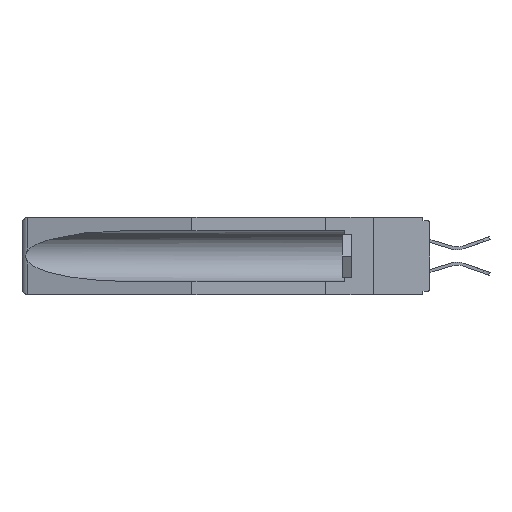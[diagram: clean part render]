
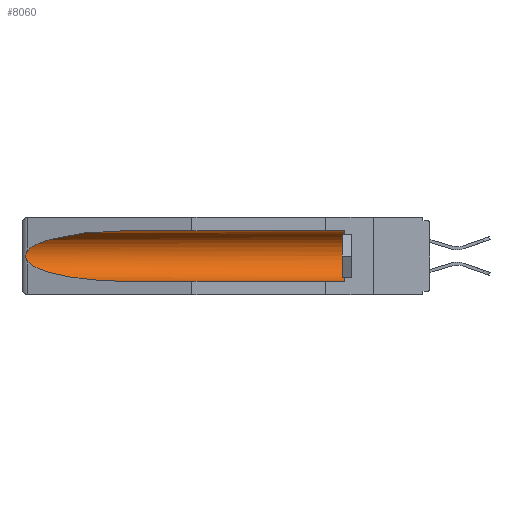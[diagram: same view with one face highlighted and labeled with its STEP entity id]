
A CAD part, left-side view. The second image highlights one B-rep face of the part: STEP entity #8060.
In plain terms, the highlighted cylindrical face has radius 2.857 mm (diameter 5.715 mm), a partial arc.
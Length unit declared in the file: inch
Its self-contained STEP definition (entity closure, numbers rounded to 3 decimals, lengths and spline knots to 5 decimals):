
#760 = CARTESIAN_POINT ( 'NONE',  ( 0.155, 1.07973, -0.059 ) ) ;
#1066 = EDGE_CURVE ( 'NONE', #5734, #5303, #21743, .T. ) ;
#1466 = B_SPLINE_CURVE_WITH_KNOTS ( 'NONE', 3,
 ( #27650, #20609, #22734, #22942, #6722, #8771, #11321, #1929, #9079, #29815 ),
 .UNSPECIFIED., .F., .F.,
 ( 4, 2, 2, 2, 4 ),
 ( 0., 0.00029, 0.00058, 0.00087, 0.00117 ),
 .UNSPECIFIED. ) ;
#1504 = EDGE_CURVE ( 'NONE', #16624, #14132, #22618, .T. ) ;
#1614 = DIRECTION ( 'NONE',  ( 0., 1., 0. ) ) ;
#1929 = CARTESIAN_POINT ( 'NONE',  ( 0.26655, 1.53094, -0.18657 ) ) ;
#2790 = CARTESIAN_POINT ( 'NONE',  ( 0.26537, 1.52718, -0.14972 ) ) ;
#3173 = CARTESIAN_POINT ( 'NONE',  ( 0.26537, 1.52718, -0.19328 ) ) ;
#3912 = EDGE_CURVE ( 'NONE', #19961, #5734, #8403, .T. ) ;
#4807 = CARTESIAN_POINT ( 'NONE',  ( 0.26537, 1.52718, -0.19328 ) ) ;
#5166 = EDGE_CURVE ( 'NONE', #19964, #16624, #1466, .T. ) ;
#5303 = VERTEX_POINT ( 'NONE', #760 ) ;
#5704 = EDGE_CURVE ( 'NONE', #5303, #19964, #9924, .T. ) ;
#5734 = VERTEX_POINT ( 'NONE', #8223 ) ;
#5757 = DIRECTION ( 'NONE',  ( 0., 0., 1. ) ) ;
#6722 = CARTESIAN_POINT ( 'NONE',  ( 0.2675, 1.53308, -0.16763 ) ) ;
#6724 = DIRECTION ( 'NONE',  ( 0., 0., 1. ) ) ;
#6966 = EDGE_CURVE ( 'NONE', #19961, #14132, #21875, .T. ) ;
#7231 = CARTESIAN_POINT ( 'NONE',  ( 0.21114, 1.30732, -0.059 ) ) ;
#8060 = ADVANCED_FACE ( 'NONE', ( #22507 ), #10118, .F. ) ;
#8223 = CARTESIAN_POINT ( 'NONE',  ( 0.155, 0.126, -0.059 ) ) ;
#8403 = CIRCLE ( 'NONE', #21635, 0.1125 ) ;
#8771 = CARTESIAN_POINT ( 'NONE',  ( 0.2675, 1.53308, -0.17534 ) ) ;
#9065 = DIRECTION ( 'NONE',  ( 0., 1., 0. ) ) ;
#9079 = CARTESIAN_POINT ( 'NONE',  ( 0.26597, 1.5296, -0.19026 ) ) ;
#9643 = CARTESIAN_POINT ( 'NONE',  ( 0.25451, 1.48313, -0.24835 ) ) ;
#9924 =( BOUNDED_CURVE ( )  B_SPLINE_CURVE ( 3, ( #13668, #7231, #25914, #14076 ),
 .UNSPECIFIED., .F., .F. ) 
 B_SPLINE_CURVE_WITH_KNOTS ( ( 4, 4 ),
 ( 4.71239, 6.08839 ),
 .UNSPECIFIED. ) 
 CURVE ( )  GEOMETRIC_REPRESENTATION_ITEM ( )  RATIONAL_B_SPLINE_CURVE ( ( 1., 0.848, 0.848, 1. ) ) 
 REPRESENTATION_ITEM ( '' )  );
#10118 = CYLINDRICAL_SURFACE ( 'NONE', #18815, 0.1125 ) ;
#11321 = CARTESIAN_POINT ( 'NONE',  ( 0.2673, 1.53269, -0.17917 ) ) ;
#12942 = DIRECTION ( 'NONE',  ( 0., 1., 0. ) ) ;
#13277 = ORIENTED_EDGE ( 'NONE', *, *, #1504, .T. ) ;
#13668 = CARTESIAN_POINT ( 'NONE',  ( 0.155, 1.07973, -0.059 ) ) ;
#13702 = VECTOR ( 'NONE', #9065, 39.37008 ) ;
#14076 = CARTESIAN_POINT ( 'NONE',  ( 0.26537, 1.52718, -0.14972 ) ) ;
#14132 = VERTEX_POINT ( 'NONE', #18779 ) ;
#14437 = CARTESIAN_POINT ( 'NONE',  ( 0.155, 1.07973, -0.284 ) ) ;
#14639 = ORIENTED_EDGE ( 'NONE', *, *, #1066, .T. ) ;
#15989 = CARTESIAN_POINT ( 'NONE',  ( 0.155, -0.30754, -0.059 ) ) ;
#16254 = ORIENTED_EDGE ( 'NONE', *, *, #5166, .T. ) ;
#16589 = CARTESIAN_POINT ( 'NONE',  ( 0.155, 0.126, -0.284 ) ) ;
#16624 = VERTEX_POINT ( 'NONE', #3173 ) ;
#18779 = CARTESIAN_POINT ( 'NONE',  ( 0.155, 1.07973, -0.284 ) ) ;
#18815 = AXIS2_PLACEMENT_3D ( 'NONE', #25103, #1614, #6724 ) ;
#19131 = CARTESIAN_POINT ( 'NONE',  ( 0.155, -0.30754, -0.284 ) ) ;
#19487 = ORIENTED_EDGE ( 'NONE', *, *, #3912, .T. ) ;
#19795 = CARTESIAN_POINT ( 'NONE',  ( 0.155, 0.126, -0.1715 ) ) ;
#19961 = VERTEX_POINT ( 'NONE', #16589 ) ;
#19964 = VERTEX_POINT ( 'NONE', #2790 ) ;
#20609 = CARTESIAN_POINT ( 'NONE',  ( 0.26597, 1.52961, -0.15275 ) ) ;
#21169 = CARTESIAN_POINT ( 'NONE',  ( 0.21114, 1.30732, -0.284 ) ) ;
#21635 = AXIS2_PLACEMENT_3D ( 'NONE', #19795, #21798, #5757 ) ;
#21743 = LINE ( 'NONE', #15989, #13702 ) ;
#21798 = DIRECTION ( 'NONE',  ( 0., -1., 0. ) ) ;
#21875 = LINE ( 'NONE', #19131, #27733 ) ;
#22507 = FACE_OUTER_BOUND ( 'NONE', #24302, .T. ) ;
#22618 =( BOUNDED_CURVE ( )  B_SPLINE_CURVE ( 3, ( #4807, #9643, #21169, #14437 ),
 .UNSPECIFIED., .F., .F. ) 
 B_SPLINE_CURVE_WITH_KNOTS ( ( 4, 4 ),
 ( 0.1948, 1.5708 ),
 .UNSPECIFIED. ) 
 CURVE ( )  GEOMETRIC_REPRESENTATION_ITEM ( )  RATIONAL_B_SPLINE_CURVE ( ( 1., 0.848, 0.848, 1. ) ) 
 REPRESENTATION_ITEM ( '' )  );
#22734 = CARTESIAN_POINT ( 'NONE',  ( 0.26654, 1.53092, -0.15636 ) ) ;
#22942 = CARTESIAN_POINT ( 'NONE',  ( 0.2673, 1.5327, -0.16383 ) ) ;
#24302 = EDGE_LOOP ( 'NONE', ( #26652, #16254, #13277, #28829, #19487, #14639 ) ) ;
#25103 = CARTESIAN_POINT ( 'NONE',  ( 0.155, -0.30754, -0.1715 ) ) ;
#25914 = CARTESIAN_POINT ( 'NONE',  ( 0.25451, 1.48313, -0.09465 ) ) ;
#26652 = ORIENTED_EDGE ( 'NONE', *, *, #5704, .T. ) ;
#27650 = CARTESIAN_POINT ( 'NONE',  ( 0.26537, 1.52718, -0.14972 ) ) ;
#27733 = VECTOR ( 'NONE', #12942, 39.37008 ) ;
#28829 = ORIENTED_EDGE ( 'NONE', *, *, #6966, .F. ) ;
#29815 = CARTESIAN_POINT ( 'NONE',  ( 0.26537, 1.52718, -0.19328 ) ) ;
